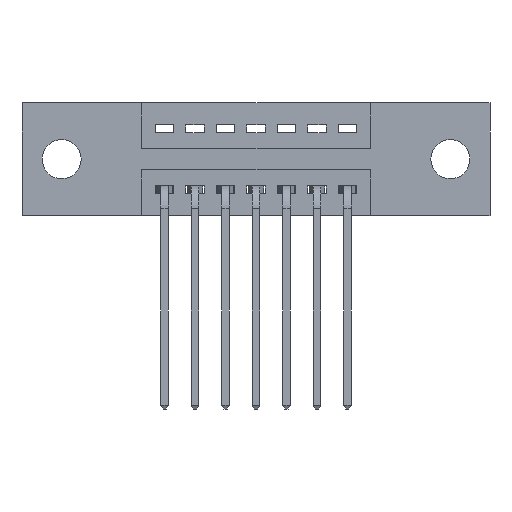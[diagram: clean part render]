
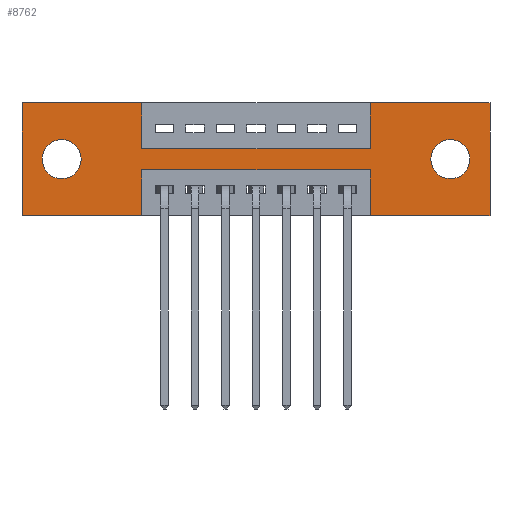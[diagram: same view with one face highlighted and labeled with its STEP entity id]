
A CAD part, front view. The second image highlights one B-rep face of the part: STEP entity #8762.
In plain terms, the highlighted planar face has unit normal (0, -1, 0).
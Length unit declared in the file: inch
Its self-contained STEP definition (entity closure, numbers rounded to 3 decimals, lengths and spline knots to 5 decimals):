
#66 = ORIENTED_EDGE ( 'NONE', *, *, #6943, .F. ) ;
#69 = VERTEX_POINT ( 'NONE', #3677 ) ;
#141 = CARTESIAN_POINT ( 'NONE',  ( 1.1425, 0., -0.37 ) ) ;
#191 = EDGE_LOOP ( 'NONE', ( #3832, #8651 ) ) ;
#304 = DIRECTION ( 'NONE',  ( 0., 0., -1. ) ) ;
#370 = DIRECTION ( 'NONE',  ( 0., 0., 1. ) ) ;
#441 = LINE ( 'NONE', #4145, #8482 ) ;
#481 = CIRCLE ( 'NONE', #8488, 0.064 ) ;
#501 = LINE ( 'NONE', #3461, #3161 ) ;
#515 = EDGE_CURVE ( 'NONE', #5115, #1858, #6618, .T. ) ;
#819 = DIRECTION ( 'NONE',  ( 0., 0., -1. ) ) ;
#824 = EDGE_CURVE ( 'NONE', #9131, #8453, #8676, .T. ) ;
#848 = CARTESIAN_POINT ( 'NONE',  ( 0., 0., -0.37 ) ) ;
#1033 = VERTEX_POINT ( 'NONE', #9402 ) ;
#1111 = EDGE_CURVE ( 'NONE', #7861, #9131, #1115, .T. ) ;
#1115 = LINE ( 'NONE', #2588, #4516 ) ;
#1331 = ORIENTED_EDGE ( 'NONE', *, *, #6203, .T. ) ;
#1480 = VECTOR ( 'NONE', #5248, 39.37008 ) ;
#1486 = CARTESIAN_POINT ( 'NONE',  ( 1.405, 0., -0.185 ) ) ;
#1583 = LINE ( 'NONE', #2135, #2658 ) ;
#1587 = CARTESIAN_POINT ( 'NONE',  ( 0.3925, 0., -0.15 ) ) ;
#1646 = LINE ( 'NONE', #3482, #3720 ) ;
#1735 = CARTESIAN_POINT ( 'NONE',  ( 0.3925, 0., -0.37 ) ) ;
#1759 = ORIENTED_EDGE ( 'NONE', *, *, #6229, .F. ) ;
#1830 = LINE ( 'NONE', #8129, #5251 ) ;
#1858 = VERTEX_POINT ( 'NONE', #8478 ) ;
#1926 = AXIS2_PLACEMENT_3D ( 'NONE', #7170, #3305, #4894 ) ;
#1968 = VECTOR ( 'NONE', #3146, 39.37008 ) ;
#2037 = CARTESIAN_POINT ( 'NONE',  ( 0., 0., -0.37 ) ) ;
#2072 = EDGE_CURVE ( 'NONE', #6483, #2522, #1830, .T. ) ;
#2135 = CARTESIAN_POINT ( 'NONE',  ( 0., 0., 0. ) ) ;
#2171 = ORIENTED_EDGE ( 'NONE', *, *, #515, .F. ) ;
#2337 = EDGE_CURVE ( 'NONE', #9544, #8695, #3775, .T. ) ;
#2361 = CARTESIAN_POINT ( 'NONE',  ( 0., 0., -0.37 ) ) ;
#2379 = EDGE_CURVE ( 'NONE', #1033, #3652, #481, .T. ) ;
#2422 = EDGE_CURVE ( 'NONE', #4653, #6483, #8254, .T. ) ;
#2522 = VERTEX_POINT ( 'NONE', #7972 ) ;
#2525 = LINE ( 'NONE', #6132, #2901 ) ;
#2526 = ORIENTED_EDGE ( 'NONE', *, *, #2337, .T. ) ;
#2528 = CARTESIAN_POINT ( 'NONE',  ( 0.3925, 0., 0. ) ) ;
#2588 = CARTESIAN_POINT ( 'NONE',  ( 1.1425, 0., 0. ) ) ;
#2658 = VECTOR ( 'NONE', #9136, 39.37008 ) ;
#2714 = EDGE_LOOP ( 'NONE', ( #1331, #2526 ) ) ;
#2901 = VECTOR ( 'NONE', #9432, 39.37008 ) ;
#2908 = EDGE_CURVE ( 'NONE', #1858, #69, #8342, .T. ) ;
#3094 = EDGE_CURVE ( 'NONE', #8453, #4653, #441, .T. ) ;
#3138 = DIRECTION ( 'NONE',  ( 0., 0., 1. ) ) ;
#3146 = DIRECTION ( 'NONE',  ( 1., 0., 0. ) ) ;
#3161 = VECTOR ( 'NONE', #6574, 39.37008 ) ;
#3252 = EDGE_CURVE ( 'NONE', #2522, #5115, #1646, .T. ) ;
#3255 = CIRCLE ( 'NONE', #3417, 0.064 ) ;
#3286 = CIRCLE ( 'NONE', #1926, 0.064 ) ;
#3305 = DIRECTION ( 'NONE',  ( 0., 1., 0. ) ) ;
#3372 = FACE_BOUND ( 'NONE', #191, .T. ) ;
#3392 = CARTESIAN_POINT ( 'NONE',  ( 0.13, 0., -0.185 ) ) ;
#3417 = AXIS2_PLACEMENT_3D ( 'NONE', #3392, #8913, #7306 ) ;
#3461 = CARTESIAN_POINT ( 'NONE',  ( 0., 0., 0. ) ) ;
#3482 = CARTESIAN_POINT ( 'NONE',  ( 0.3925, 0., -0.22 ) ) ;
#3507 = DIRECTION ( 'NONE',  ( -1., 0., 0. ) ) ;
#3652 = VERTEX_POINT ( 'NONE', #5710 ) ;
#3677 = CARTESIAN_POINT ( 'NONE',  ( 0., 0., -0.37 ) ) ;
#3720 = VECTOR ( 'NONE', #3507, 39.37008 ) ;
#3775 = CIRCLE ( 'NONE', #7957, 0.064 ) ;
#3832 = ORIENTED_EDGE ( 'NONE', *, *, #7365, .T. ) ;
#3850 = ORIENTED_EDGE ( 'NONE', *, *, #2072, .F. ) ;
#3896 = CARTESIAN_POINT ( 'NONE',  ( 0., 0., 0. ) ) ;
#4019 = CARTESIAN_POINT ( 'NONE',  ( 0.13, 0., -0.185 ) ) ;
#4142 = DIRECTION ( 'NONE',  ( 0., 0., 1. ) ) ;
#4145 = CARTESIAN_POINT ( 'NONE',  ( 1.535, 0., 0. ) ) ;
#4516 = VECTOR ( 'NONE', #4142, 39.37008 ) ;
#4620 = DIRECTION ( 'NONE',  ( 0., 1., 0. ) ) ;
#4621 = VECTOR ( 'NONE', #7777, 39.37008 ) ;
#4653 = VERTEX_POINT ( 'NONE', #9303 ) ;
#4815 = CARTESIAN_POINT ( 'NONE',  ( 1.535, 0., 0. ) ) ;
#4894 = DIRECTION ( 'NONE',  ( 0., 0., -1. ) ) ;
#5115 = VERTEX_POINT ( 'NONE', #7029 ) ;
#5248 = DIRECTION ( 'NONE',  ( 1., 0., 0. ) ) ;
#5251 = VECTOR ( 'NONE', #370, 39.37008 ) ;
#5345 = CARTESIAN_POINT ( 'NONE',  ( 1.1425, 0., 0. ) ) ;
#5411 = CARTESIAN_POINT ( 'NONE',  ( 1.405, 0., -0.121 ) ) ;
#5450 = FACE_BOUND ( 'NONE', #2714, .T. ) ;
#5544 = VERTEX_POINT ( 'NONE', #2528 ) ;
#5710 = CARTESIAN_POINT ( 'NONE',  ( 0.13, 0., -0.121 ) ) ;
#5916 = EDGE_LOOP ( 'NONE', ( #2171, #6339, #3850, #7536, #8375, #8412, #8137, #1759, #6016, #9177, #66, #8632 ) ) ;
#5925 = AXIS2_PLACEMENT_3D ( 'NONE', #2361, #7883, #819 ) ;
#6016 = ORIENTED_EDGE ( 'NONE', *, *, #7544, .F. ) ;
#6132 = CARTESIAN_POINT ( 'NONE',  ( 0.3925, 0., 0. ) ) ;
#6203 = EDGE_CURVE ( 'NONE', #8695, #9544, #3286, .T. ) ;
#6229 = EDGE_CURVE ( 'NONE', #6890, #7861, #7671, .T. ) ;
#6321 = EDGE_CURVE ( 'NONE', #8951, #5544, #501, .T. ) ;
#6339 = ORIENTED_EDGE ( 'NONE', *, *, #3252, .F. ) ;
#6483 = VERTEX_POINT ( 'NONE', #141 ) ;
#6574 = DIRECTION ( 'NONE',  ( 1., 0., 0. ) ) ;
#6618 = LINE ( 'NONE', #1735, #9275 ) ;
#6882 = DIRECTION ( 'NONE',  ( 0., 0., -1. ) ) ;
#6890 = VERTEX_POINT ( 'NONE', #8974 ) ;
#6938 = FACE_OUTER_BOUND ( 'NONE', #5916, .T. ) ;
#6943 = EDGE_CURVE ( 'NONE', #69, #8951, #1583, .T. ) ;
#7029 = CARTESIAN_POINT ( 'NONE',  ( 0.3925, 0., -0.22 ) ) ;
#7170 = CARTESIAN_POINT ( 'NONE',  ( 1.405, 0., -0.185 ) ) ;
#7228 = CARTESIAN_POINT ( 'NONE',  ( 1.1425, 0., -0.15 ) ) ;
#7306 = DIRECTION ( 'NONE',  ( 0., 0., 1. ) ) ;
#7365 = EDGE_CURVE ( 'NONE', #3652, #1033, #3255, .T. ) ;
#7536 = ORIENTED_EDGE ( 'NONE', *, *, #2422, .F. ) ;
#7544 = EDGE_CURVE ( 'NONE', #5544, #6890, #2525, .T. ) ;
#7671 = LINE ( 'NONE', #1587, #1968 ) ;
#7777 = DIRECTION ( 'NONE',  ( -1., 0., 0. ) ) ;
#7855 = VECTOR ( 'NONE', #10037, 39.37008 ) ;
#7861 = VERTEX_POINT ( 'NONE', #7228 ) ;
#7883 = DIRECTION ( 'NONE',  ( 0., -1., 0. ) ) ;
#7912 = PLANE ( 'NONE',  #5925 ) ;
#7957 = AXIS2_PLACEMENT_3D ( 'NONE', #1486, #8502, #6882 ) ;
#7972 = CARTESIAN_POINT ( 'NONE',  ( 1.1425, 0., -0.22 ) ) ;
#8052 = DIRECTION ( 'NONE',  ( 0., 0., -1. ) ) ;
#8129 = CARTESIAN_POINT ( 'NONE',  ( 1.1425, 0., -0.37 ) ) ;
#8137 = ORIENTED_EDGE ( 'NONE', *, *, #1111, .F. ) ;
#8254 = LINE ( 'NONE', #848, #4621 ) ;
#8342 = LINE ( 'NONE', #2037, #7855 ) ;
#8375 = ORIENTED_EDGE ( 'NONE', *, *, #3094, .F. ) ;
#8412 = ORIENTED_EDGE ( 'NONE', *, *, #824, .F. ) ;
#8453 = VERTEX_POINT ( 'NONE', #4815 ) ;
#8478 = CARTESIAN_POINT ( 'NONE',  ( 0.3925, 0., -0.37 ) ) ;
#8482 = VECTOR ( 'NONE', #8052, 39.37008 ) ;
#8488 = AXIS2_PLACEMENT_3D ( 'NONE', #4019, #4620, #3138 ) ;
#8502 = DIRECTION ( 'NONE',  ( 0., 1., 0. ) ) ;
#8632 = ORIENTED_EDGE ( 'NONE', *, *, #2908, .F. ) ;
#8651 = ORIENTED_EDGE ( 'NONE', *, *, #2379, .T. ) ;
#8676 = LINE ( 'NONE', #9069, #1480 ) ;
#8695 = VERTEX_POINT ( 'NONE', #5411 ) ;
#8762 = ADVANCED_FACE ( 'NONE', ( #5450, #3372, #6938 ), #7912, .T. ) ;
#8913 = DIRECTION ( 'NONE',  ( 0., 1., 0. ) ) ;
#8951 = VERTEX_POINT ( 'NONE', #3896 ) ;
#8974 = CARTESIAN_POINT ( 'NONE',  ( 0.3925, 0., -0.15 ) ) ;
#9069 = CARTESIAN_POINT ( 'NONE',  ( 0., 0., 0. ) ) ;
#9131 = VERTEX_POINT ( 'NONE', #5345 ) ;
#9136 = DIRECTION ( 'NONE',  ( 0., 0., 1. ) ) ;
#9177 = ORIENTED_EDGE ( 'NONE', *, *, #6321, .F. ) ;
#9275 = VECTOR ( 'NONE', #304, 39.37008 ) ;
#9303 = CARTESIAN_POINT ( 'NONE',  ( 1.535, 0., -0.37 ) ) ;
#9336 = CARTESIAN_POINT ( 'NONE',  ( 1.405, 0., -0.249 ) ) ;
#9402 = CARTESIAN_POINT ( 'NONE',  ( 0.13, 0., -0.249 ) ) ;
#9432 = DIRECTION ( 'NONE',  ( 0., 0., -1. ) ) ;
#9544 = VERTEX_POINT ( 'NONE', #9336 ) ;
#10037 = DIRECTION ( 'NONE',  ( -1., 0., 0. ) ) ;
